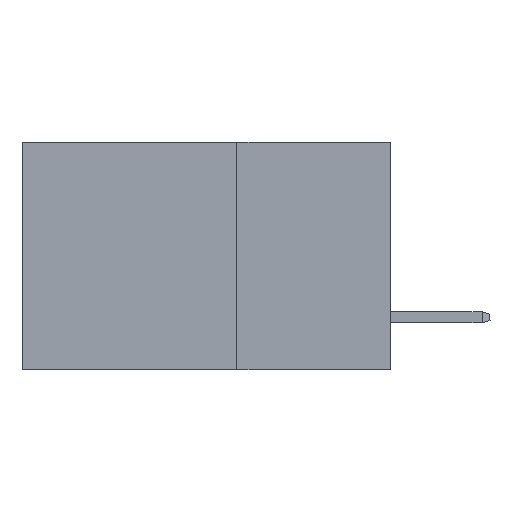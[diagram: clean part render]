
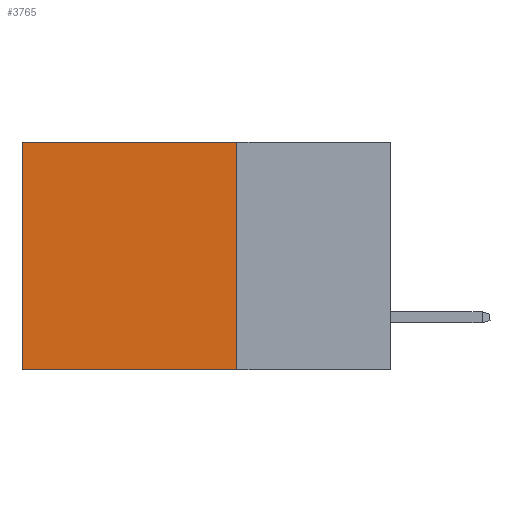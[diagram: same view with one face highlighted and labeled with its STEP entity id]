
A CAD part, left-side view. The second image highlights one B-rep face of the part: STEP entity #3765.
In plain terms, the highlighted planar face has unit normal (-1, 0, 0).
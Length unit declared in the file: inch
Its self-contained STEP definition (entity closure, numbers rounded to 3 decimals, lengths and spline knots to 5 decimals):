
#293 = CARTESIAN_POINT ( 'NONE',  ( 0.2875, 0.6, 0. ) ) ;
#475 = CARTESIAN_POINT ( 'NONE',  ( 0.2875, 0.6, 0. ) ) ;
#479 = DIRECTION ( 'NONE',  ( 0., 0., -1. ) ) ;
#614 = ORIENTED_EDGE ( 'NONE', *, *, #4477, .T. ) ;
#746 = CARTESIAN_POINT ( 'NONE',  ( 0.2875, 0.25, 0. ) ) ;
#799 = ORIENTED_EDGE ( 'NONE', *, *, #9147, .F. ) ;
#849 = ORIENTED_EDGE ( 'NONE', *, *, #2554, .F. ) ;
#975 = ORIENTED_EDGE ( 'NONE', *, *, #7031, .T. ) ;
#1007 = LINE ( 'NONE', #746, #7123 ) ;
#1200 = DIRECTION ( 'NONE',  ( 0., 1., 0. ) ) ;
#1296 = EDGE_LOOP ( 'NONE', ( #614, #799, #849, #975 ) ) ;
#1813 = CARTESIAN_POINT ( 'NONE',  ( 0.2875, 0.25, -0.37 ) ) ;
#2554 = EDGE_CURVE ( 'NONE', #3798, #6484, #3886, .T. ) ;
#3105 = DIRECTION ( 'NONE',  ( 0., 1., 0. ) ) ;
#3765 = ADVANCED_FACE ( 'NONE', ( #8267 ), #6411, .F. ) ;
#3798 = VERTEX_POINT ( 'NONE', #6159 ) ;
#3886 = LINE ( 'NONE', #9233, #7438 ) ;
#4477 = EDGE_CURVE ( 'NONE', #4937, #4898, #5667, .T. ) ;
#4606 = CARTESIAN_POINT ( 'NONE',  ( 0.2875, 0.6, -0.37 ) ) ;
#4898 = VERTEX_POINT ( 'NONE', #4606 ) ;
#4937 = VERTEX_POINT ( 'NONE', #293 ) ;
#5667 = LINE ( 'NONE', #475, #7499 ) ;
#6159 = CARTESIAN_POINT ( 'NONE',  ( 0.2875, 0.25, 0. ) ) ;
#6411 = PLANE ( 'NONE',  #7042 ) ;
#6484 = VERTEX_POINT ( 'NONE', #1813 ) ;
#7031 = EDGE_CURVE ( 'NONE', #3798, #4937, #1007, .T. ) ;
#7042 = AXIS2_PLACEMENT_3D ( 'NONE', #7162, #7045, #7090 ) ;
#7045 = DIRECTION ( 'NONE',  ( 1., 0., 0. ) ) ;
#7090 = DIRECTION ( 'NONE',  ( 0., 0., -1. ) ) ;
#7123 = VECTOR ( 'NONE', #3105, 39.37008 ) ;
#7162 = CARTESIAN_POINT ( 'NONE',  ( 0.2875, 0.25, 0. ) ) ;
#7184 = VECTOR ( 'NONE', #1200, 39.37008 ) ;
#7438 = VECTOR ( 'NONE', #9320, 39.37008 ) ;
#7499 = VECTOR ( 'NONE', #479, 39.37008 ) ;
#8267 = FACE_OUTER_BOUND ( 'NONE', #1296, .T. ) ;
#8422 = CARTESIAN_POINT ( 'NONE',  ( 0.2875, 0.25, -0.37 ) ) ;
#8955 = LINE ( 'NONE', #8422, #7184 ) ;
#9147 = EDGE_CURVE ( 'NONE', #6484, #4898, #8955, .T. ) ;
#9233 = CARTESIAN_POINT ( 'NONE',  ( 0.2875, 0.25, 0. ) ) ;
#9320 = DIRECTION ( 'NONE',  ( 0., 0., -1. ) ) ;
